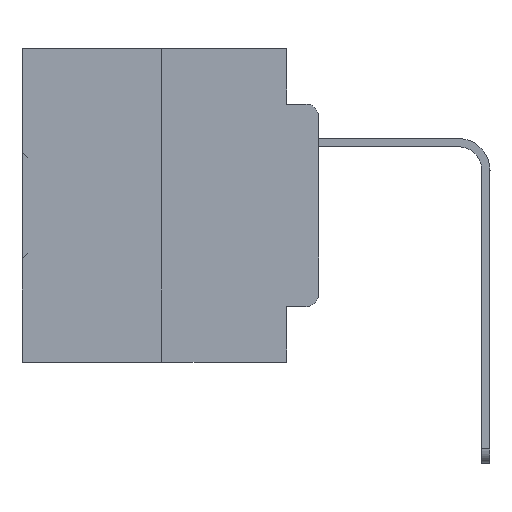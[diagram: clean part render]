
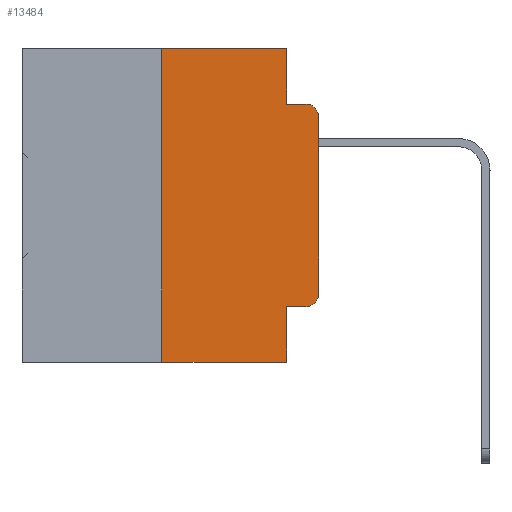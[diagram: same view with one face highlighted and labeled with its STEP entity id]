
A CAD part, left-side view. The second image highlights one B-rep face of the part: STEP entity #13484.
In plain terms, the highlighted planar face has unit normal (-1, 0, 0).
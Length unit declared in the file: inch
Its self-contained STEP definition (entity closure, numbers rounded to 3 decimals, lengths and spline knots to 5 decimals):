
#205 = CARTESIAN_POINT ( 'NONE',  ( 0., 0., -0.1085 ) ) ;
#259 = LINE ( 'NONE', #34721, #6601 ) ;
#355 = DIRECTION ( 'NONE',  ( 0., -1., 0. ) ) ;
#368 = LINE ( 'NONE', #8390, #3345 ) ;
#452 = CARTESIAN_POINT ( 'NONE',  ( 0., 0.02, -0.0885 ) ) ;
#490 = CARTESIAN_POINT ( 'NONE',  ( 0., 0.051, 0. ) ) ;
#1598 = VERTEX_POINT ( 'NONE', #3697 ) ;
#1648 = DIRECTION ( 'NONE',  ( 1., 0., 0. ) ) ;
#1824 = CARTESIAN_POINT ( 'NONE',  ( 0., 0., -0.3915 ) ) ;
#1929 = DIRECTION ( 'NONE',  ( 0., 0., -1. ) ) ;
#2384 = DIRECTION ( 'NONE',  ( 0., -1., 0. ) ) ;
#2655 = DIRECTION ( 'NONE',  ( 0., 0., -1. ) ) ;
#3088 = EDGE_CURVE ( 'NONE', #24478, #29987, #259, .T. ) ;
#3260 = EDGE_LOOP ( 'NONE', ( #22404, #35026, #5233, #29741, #14810, #25151, #14729, #3840, #15104, #7427 ) ) ;
#3345 = VECTOR ( 'NONE', #355, 39.37008 ) ;
#3697 = CARTESIAN_POINT ( 'NONE',  ( 0., 0.051, -0.4115 ) ) ;
#3840 = ORIENTED_EDGE ( 'NONE', *, *, #26506, .F. ) ;
#4076 = VERTEX_POINT ( 'NONE', #20797 ) ;
#4171 = FACE_OUTER_BOUND ( 'NONE', #3260, .T. ) ;
#4425 = LINE ( 'NONE', #5786, #21370 ) ;
#4648 = CARTESIAN_POINT ( 'NONE',  ( 0., 0.051, -0.4115 ) ) ;
#4977 = CARTESIAN_POINT ( 'NONE',  ( 0., 0.02, -0.4115 ) ) ;
#5233 = ORIENTED_EDGE ( 'NONE', *, *, #23648, .F. ) ;
#5786 = CARTESIAN_POINT ( 'NONE',  ( 0., 0.051, 0. ) ) ;
#6343 = VERTEX_POINT ( 'NONE', #18235 ) ;
#6601 = VECTOR ( 'NONE', #24115, 39.37008 ) ;
#7274 = CARTESIAN_POINT ( 'NONE',  ( 0., 0.051, -0.5 ) ) ;
#7357 = DIRECTION ( 'NONE',  ( -1., 0., 0. ) ) ;
#7427 = ORIENTED_EDGE ( 'NONE', *, *, #7738, .T. ) ;
#7738 = EDGE_CURVE ( 'NONE', #8511, #24478, #30226, .T. ) ;
#8307 = CARTESIAN_POINT ( 'NONE',  ( 0., 0.02, -0.1085 ) ) ;
#8390 = CARTESIAN_POINT ( 'NONE',  ( 0., 0.051, -0.0885 ) ) ;
#8511 = VERTEX_POINT ( 'NONE', #4977 ) ;
#8898 = VECTOR ( 'NONE', #11038, 39.37008 ) ;
#9451 = EDGE_CURVE ( 'NONE', #27013, #19067, #21701, .T. ) ;
#10024 = PLANE ( 'NONE',  #32458 ) ;
#10813 = CARTESIAN_POINT ( 'NONE',  ( 0., 0.25, -0.5 ) ) ;
#11038 = DIRECTION ( 'NONE',  ( 0., -1., 0. ) ) ;
#12839 = VERTEX_POINT ( 'NONE', #452 ) ;
#13484 = ADVANCED_FACE ( 'NONE', ( #4171 ), #10024, .F. ) ;
#14484 = VECTOR ( 'NONE', #28072, 39.37008 ) ;
#14729 = ORIENTED_EDGE ( 'NONE', *, *, #28131, .T. ) ;
#14802 = LINE ( 'NONE', #16029, #8898 ) ;
#14810 = ORIENTED_EDGE ( 'NONE', *, *, #28808, .F. ) ;
#15104 = ORIENTED_EDGE ( 'NONE', *, *, #33029, .T. ) ;
#15118 = CARTESIAN_POINT ( 'NONE',  ( 0., 0.25, 0. ) ) ;
#15363 = DIRECTION ( 'NONE',  ( 0., 0., -1. ) ) ;
#15985 = VERTEX_POINT ( 'NONE', #7274 ) ;
#16029 = CARTESIAN_POINT ( 'NONE',  ( 0., 0.473, 0. ) ) ;
#17624 = AXIS2_PLACEMENT_3D ( 'NONE', #21121, #7357, #1929 ) ;
#18235 = CARTESIAN_POINT ( 'NONE',  ( 0., 0.051, 0. ) ) ;
#18478 = VECTOR ( 'NONE', #2384, 39.37008 ) ;
#18972 = DIRECTION ( 'NONE',  ( 0., 0., -1. ) ) ;
#19067 = VERTEX_POINT ( 'NONE', #15118 ) ;
#19297 = DIRECTION ( 'NONE',  ( 0., 0., -1. ) ) ;
#20797 = CARTESIAN_POINT ( 'NONE',  ( 0., 0.051, -0.0885 ) ) ;
#21121 = CARTESIAN_POINT ( 'NONE',  ( 0., 0.02, -0.3915 ) ) ;
#21370 = VECTOR ( 'NONE', #19297, 39.37008 ) ;
#21701 = LINE ( 'NONE', #31032, #14484 ) ;
#22104 = VECTOR ( 'NONE', #27163, 39.37008 ) ;
#22404 = ORIENTED_EDGE ( 'NONE', *, *, #3088, .T. ) ;
#22516 = LINE ( 'NONE', #29656, #22104 ) ;
#23648 = EDGE_CURVE ( 'NONE', #4076, #12839, #368, .T. ) ;
#24115 = DIRECTION ( 'NONE',  ( 0., 0., 1. ) ) ;
#24428 = DIRECTION ( 'NONE',  ( -1., 0., 0. ) ) ;
#24478 = VERTEX_POINT ( 'NONE', #1824 ) ;
#25151 = ORIENTED_EDGE ( 'NONE', *, *, #9451, .F. ) ;
#25882 = CARTESIAN_POINT ( 'NONE',  ( 0., 0.473, 0. ) ) ;
#26289 = AXIS2_PLACEMENT_3D ( 'NONE', #8307, #24428, #2655 ) ;
#26487 = CIRCLE ( 'NONE', #26289, 0.02 ) ;
#26506 = EDGE_CURVE ( 'NONE', #1598, #15985, #4425, .T. ) ;
#27013 = VERTEX_POINT ( 'NONE', #10813 ) ;
#27163 = DIRECTION ( 'NONE',  ( 0., -1., 0. ) ) ;
#28072 = DIRECTION ( 'NONE',  ( 0., 0., 1. ) ) ;
#28131 = EDGE_CURVE ( 'NONE', #27013, #15985, #22516, .T. ) ;
#28619 = LINE ( 'NONE', #4648, #18478 ) ;
#28808 = EDGE_CURVE ( 'NONE', #19067, #6343, #14802, .T. ) ;
#29328 = EDGE_CURVE ( 'NONE', #6343, #4076, #34630, .T. ) ;
#29656 = CARTESIAN_POINT ( 'NONE',  ( 0., 0.473, -0.5 ) ) ;
#29741 = ORIENTED_EDGE ( 'NONE', *, *, #29328, .F. ) ;
#29987 = VERTEX_POINT ( 'NONE', #205 ) ;
#30012 = VECTOR ( 'NONE', #18972, 39.37008 ) ;
#30226 = CIRCLE ( 'NONE', #17624, 0.02 ) ;
#30792 = EDGE_CURVE ( 'NONE', #29987, #12839, #26487, .T. ) ;
#31032 = CARTESIAN_POINT ( 'NONE',  ( 0., 0.25, 0. ) ) ;
#32458 = AXIS2_PLACEMENT_3D ( 'NONE', #25882, #1648, #15363 ) ;
#33029 = EDGE_CURVE ( 'NONE', #1598, #8511, #28619, .T. ) ;
#34630 = LINE ( 'NONE', #490, #30012 ) ;
#34721 = CARTESIAN_POINT ( 'NONE',  ( 0., 0., 0. ) ) ;
#35026 = ORIENTED_EDGE ( 'NONE', *, *, #30792, .T. ) ;
